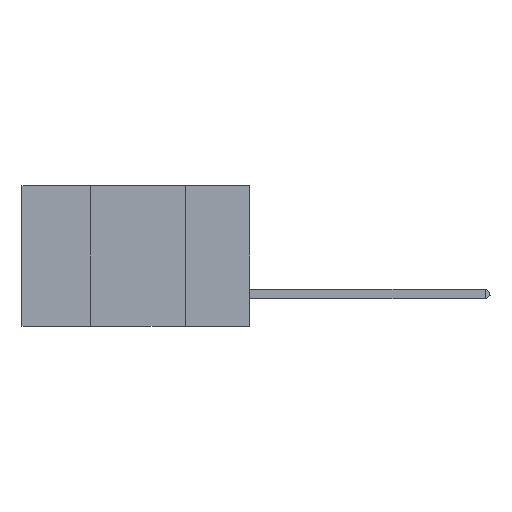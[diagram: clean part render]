
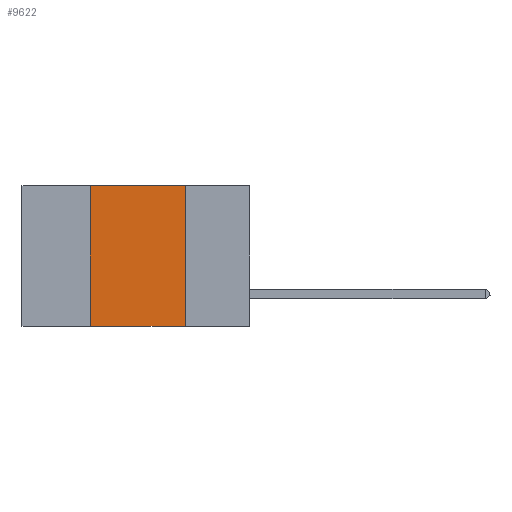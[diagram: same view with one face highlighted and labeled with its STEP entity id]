
A CAD part, left-side view. The second image highlights one B-rep face of the part: STEP entity #9622.
In plain terms, the highlighted planar face has unit normal (-1, 0, 0).
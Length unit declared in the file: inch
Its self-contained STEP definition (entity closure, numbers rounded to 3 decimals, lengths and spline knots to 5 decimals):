
#79 = CARTESIAN_POINT ( 'NONE',  ( 0., 0.42, -0.37 ) ) ;
#574 = CARTESIAN_POINT ( 'NONE',  ( 0., 0.17, -0.37 ) ) ;
#1144 = LINE ( 'NONE', #3167, #1786 ) ;
#1171 = EDGE_CURVE ( 'NONE', #10508, #9298, #6170, .T. ) ;
#1264 = EDGE_CURVE ( 'NONE', #10508, #5564, #1144, .T. ) ;
#1533 = VECTOR ( 'NONE', #2605, 39.37008 ) ;
#1580 = LINE ( 'NONE', #4371, #6347 ) ;
#1786 = VECTOR ( 'NONE', #9799, 39.37008 ) ;
#1912 = DIRECTION ( 'NONE',  ( 0., -1., 0. ) ) ;
#2214 = LINE ( 'NONE', #5284, #9962 ) ;
#2605 = DIRECTION ( 'NONE',  ( 0., 0., 1. ) ) ;
#2999 = DIRECTION ( 'NONE',  ( 1., 0., 0. ) ) ;
#3167 = CARTESIAN_POINT ( 'NONE',  ( 0., 0.6, -0.37 ) ) ;
#3800 = PLANE ( 'NONE',  #7033 ) ;
#4138 = ORIENTED_EDGE ( 'NONE', *, *, #1171, .F. ) ;
#4371 = CARTESIAN_POINT ( 'NONE',  ( 0., 0.6, 0. ) ) ;
#5284 = CARTESIAN_POINT ( 'NONE',  ( 0., 0.17, 0. ) ) ;
#5385 = CARTESIAN_POINT ( 'NONE',  ( 0., 0.17, 0. ) ) ;
#5564 = VERTEX_POINT ( 'NONE', #574 ) ;
#5568 = ORIENTED_EDGE ( 'NONE', *, *, #1264, .T. ) ;
#5915 = CARTESIAN_POINT ( 'NONE',  ( 0., 0.42, 0. ) ) ;
#5993 = DIRECTION ( 'NONE',  ( 0., 0., -1. ) ) ;
#6170 = LINE ( 'NONE', #5915, #1533 ) ;
#6347 = VECTOR ( 'NONE', #1912, 39.37008 ) ;
#6443 = ORIENTED_EDGE ( 'NONE', *, *, #10611, .F. ) ;
#6637 = ORIENTED_EDGE ( 'NONE', *, *, #9985, .F. ) ;
#7033 = AXIS2_PLACEMENT_3D ( 'NONE', #7946, #2999, #9623 ) ;
#7144 = VERTEX_POINT ( 'NONE', #5385 ) ;
#7946 = CARTESIAN_POINT ( 'NONE',  ( 0., 0.6, 0. ) ) ;
#9087 = FACE_OUTER_BOUND ( 'NONE', #10298, .T. ) ;
#9298 = VERTEX_POINT ( 'NONE', #10057 ) ;
#9622 = ADVANCED_FACE ( 'NONE', ( #9087 ), #3800, .F. ) ;
#9623 = DIRECTION ( 'NONE',  ( 0., 0., -1. ) ) ;
#9799 = DIRECTION ( 'NONE',  ( 0., -1., 0. ) ) ;
#9962 = VECTOR ( 'NONE', #5993, 39.37008 ) ;
#9985 = EDGE_CURVE ( 'NONE', #9298, #7144, #1580, .T. ) ;
#10057 = CARTESIAN_POINT ( 'NONE',  ( 0., 0.42, 0. ) ) ;
#10298 = EDGE_LOOP ( 'NONE', ( #6443, #6637, #4138, #5568 ) ) ;
#10508 = VERTEX_POINT ( 'NONE', #79 ) ;
#10611 = EDGE_CURVE ( 'NONE', #7144, #5564, #2214, .T. ) ;
